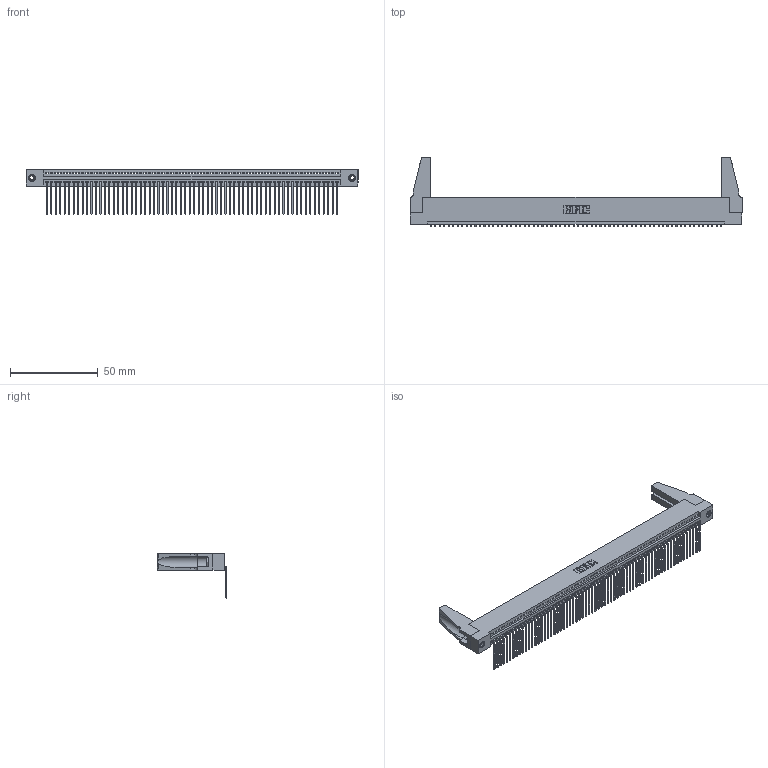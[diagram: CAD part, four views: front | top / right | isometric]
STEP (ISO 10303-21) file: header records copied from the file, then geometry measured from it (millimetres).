
FILE_DESCRIPTION (( 'STEP AP203' ), '1' );
FILE_NAME ('395-066-559-188.STEP', '2019-10-25T10:08:26', ( '' ), ( '' ), 'SwSTEP 2.0', 'SolidWorks 2016', '' );
FILE_SCHEMA (( 'CONFIG_CONTROL_DESIGN' ));
Length unit declared in the file: inch
Products named in the file (5): 345-292-001_558 559 Tail - 1; 345-220-078_345-220-088; 345-250-001_345-250-001-102; 345 Part_Flush Mounting Lugs - 0.156 Dia-TH; 395-066-559-188
Assembly tree (71 placements, depth 2):
  395-066-559-188
    345 Part_Flush Mounting Lugs - 0.156 Dia-TH
    345-292-001_558 559 Tail - 1  x66
    345-250-001_345-250-001-102  x2
    345-220-078_345-220-088  x2
Bounding box: 188.87 x 39.61 x 25.53 mm (x, y, z)
Volume: 21608.5 mm3; surface area: 29141 mm2
Topology: 71 solids, 71 shells, 4210 faces, 12667 edges, 8346 vertices
Faces by surface type: plane 2924, cylinder 1270, cone 12, torus 4
Entity records: 48674 total; most frequent: CARTESIAN_POINT 8420, ORIENTED_EDGE 8380, DIRECTION 7326, EDGE_CURVE 4190, LINE 3752, VECTOR 3752, VERTEX_POINT 2786, AXIS2_PLACEMENT_3D 1787
